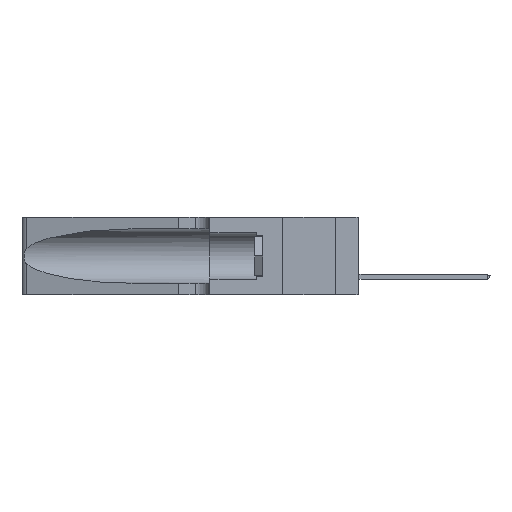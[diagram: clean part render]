
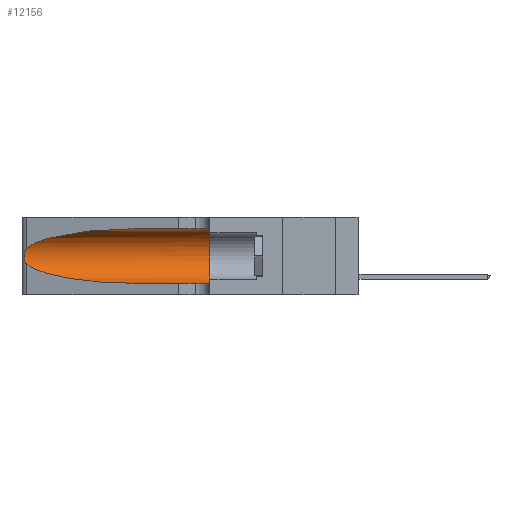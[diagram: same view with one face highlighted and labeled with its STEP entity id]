
A CAD part, left-side view. The second image highlights one B-rep face of the part: STEP entity #12156.
In plain terms, the highlighted cylindrical face has radius 3.308 mm (diameter 6.617 mm), a partial arc.
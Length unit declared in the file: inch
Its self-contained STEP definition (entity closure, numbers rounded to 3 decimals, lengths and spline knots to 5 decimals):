
#287 = B_SPLINE_CURVE_WITH_KNOTS ( 'NONE', 3,
 ( #22355, #33885, #36813, #13155, #19237, #19104, #28234, #21798, #3859, #10048, #34020, #1123, #4136, #34168 ),
 .UNSPECIFIED., .F., .F.,
 ( 4, 2, 2, 2, 2, 2, 4 ),
 ( 0., 0.00027, 0.00053, 0.00107, 0.0016, 0.00187, 0.00214 ),
 .UNSPECIFIED. ) ;
#646 = EDGE_CURVE ( 'NONE', #30015, #37181, #14277, .T. ) ;
#689 = CARTESIAN_POINT ( 'NONE',  ( 0.1305, 0.72297, 0.31525 ) ) ;
#1123 = CARTESIAN_POINT ( 'NONE',  ( 0.25639, 1.23186, 0.15144 ) ) ;
#1220 = CARTESIAN_POINT ( 'NONE',  ( 0.1305, 1.61858, 0.185 ) ) ;
#1498 = CARTESIAN_POINT ( 'NONE',  ( 0.1305, 1.61858, 0.31525 ) ) ;
#2928 = EDGE_CURVE ( 'NONE', #7715, #30015, #287, .T. ) ;
#3859 = CARTESIAN_POINT ( 'NONE',  ( 0.26017, 1.23833, 0.17102 ) ) ;
#4136 = CARTESIAN_POINT ( 'NONE',  ( 0.25555, 1.22993, 0.14849 ) ) ;
#4545 = CARTESIAN_POINT ( 'NONE',  ( 0.1305, 0.72297, 0.05475 ) ) ;
#4835 = LINE ( 'NONE', #1498, #13749 ) ;
#5540 = VERTEX_POINT ( 'NONE', #19862 ) ;
#5572 = VECTOR ( 'NONE', #37356, 39.37008 ) ;
#5904 = CARTESIAN_POINT ( 'NONE',  ( 0.25487, 1.22718, 0.22369 ) ) ;
#6229 = CARTESIAN_POINT ( 'NONE',  ( 0.25487, 1.22718, 0.14631 ) ) ;
#6385 = AXIS2_PLACEMENT_3D ( 'NONE', #1220, #34538, #34395 ) ;
#7013 = CARTESIAN_POINT ( 'NONE',  ( 0.25487, 1.22718, 0.22369 ) ) ;
#7155 = CARTESIAN_POINT ( 'NONE',  ( 0.2373, 1.15595, 0.28018 ) ) ;
#7715 = VERTEX_POINT ( 'NONE', #5904 ) ;
#8183 = ORIENTED_EDGE ( 'NONE', *, *, #2928, .T. ) ;
#8356 = CYLINDRICAL_SURFACE ( 'NONE', #6385, 0.13025 ) ;
#9649 = FACE_OUTER_BOUND ( 'NONE', #17999, .T. ) ;
#10024 = DIRECTION ( 'NONE',  ( 0., -1., 0. ) ) ;
#10048 = CARTESIAN_POINT ( 'NONE',  ( 0.25856, 1.23593, 0.16098 ) ) ;
#10107 = CARTESIAN_POINT ( 'NONE',  ( 0.1305, 0.35, 0.185 ) ) ;
#10376 = DIRECTION ( 'NONE',  ( 0., 1., 0. ) ) ;
#10422 = EDGE_CURVE ( 'NONE', #11902, #5540, #28086, .T. ) ;
#10718 = CARTESIAN_POINT ( 'NONE',  ( 0.2373, 1.15595, 0.08982 ) ) ;
#11196 = CARTESIAN_POINT ( 'NONE',  ( 0.1305, 0.72297, 0.05475 ) ) ;
#11902 = VERTEX_POINT ( 'NONE', #19878 ) ;
#12156 = ADVANCED_FACE ( 'NONE', ( #9649 ), #8356, .F. ) ;
#13155 = CARTESIAN_POINT ( 'NONE',  ( 0.25787, 1.23484, 0.2124 ) ) ;
#13441 = ORIENTED_EDGE ( 'NONE', *, *, #10422, .F. ) ;
#13749 = VECTOR ( 'NONE', #10024, 39.37008 ) ;
#14277 =( BOUNDED_CURVE ( )  B_SPLINE_CURVE ( 3, ( #31507, #10718, #31638, #4545 ),
 .UNSPECIFIED., .F., .T. ) 
 B_SPLINE_CURVE_WITH_KNOTS ( ( 4, 4 ),
 ( 3.44316, 4.71239 ),
 .UNSPECIFIED. ) 
 CURVE ( )  GEOMETRIC_REPRESENTATION_ITEM ( )  RATIONAL_B_SPLINE_CURVE ( ( 1., 0.87, 0.87, 1. ) ) 
 REPRESENTATION_ITEM ( '' )  );
#15396 =( BOUNDED_CURVE ( )  B_SPLINE_CURVE ( 3, ( #689, #18948, #7155, #7013 ),
 .UNSPECIFIED., .F., .T. ) 
 B_SPLINE_CURVE_WITH_KNOTS ( ( 4, 4 ),
 ( 1.5708, 2.84003 ),
 .UNSPECIFIED. ) 
 CURVE ( )  GEOMETRIC_REPRESENTATION_ITEM ( )  RATIONAL_B_SPLINE_CURVE ( ( 1., 0.87, 0.87, 1. ) ) 
 REPRESENTATION_ITEM ( '' )  );
#16196 = VERTEX_POINT ( 'NONE', #25013 ) ;
#16547 = EDGE_CURVE ( 'NONE', #37181, #5540, #37481, .T. ) ;
#16785 = EDGE_CURVE ( 'NONE', #16196, #7715, #15396, .T. ) ;
#17999 = EDGE_LOOP ( 'NONE', ( #30331, #8183, #38618, #18238, #13441, #19939 ) ) ;
#18238 = ORIENTED_EDGE ( 'NONE', *, *, #16547, .T. ) ;
#18948 = CARTESIAN_POINT ( 'NONE',  ( 0.18966, 0.96281, 0.31525 ) ) ;
#19104 = CARTESIAN_POINT ( 'NONE',  ( 0.26018, 1.23835, 0.19895 ) ) ;
#19237 = CARTESIAN_POINT ( 'NONE',  ( 0.25854, 1.2359, 0.20912 ) ) ;
#19862 = CARTESIAN_POINT ( 'NONE',  ( 0.1305, 0.35, 0.05475 ) ) ;
#19878 = CARTESIAN_POINT ( 'NONE',  ( 0.1305, 0.35, 0.31525 ) ) ;
#19939 = ORIENTED_EDGE ( 'NONE', *, *, #29448, .F. ) ;
#21798 = CARTESIAN_POINT ( 'NONE',  ( 0.26075, 1.23896, 0.178 ) ) ;
#22355 = CARTESIAN_POINT ( 'NONE',  ( 0.25487, 1.22718, 0.22369 ) ) ;
#25013 = CARTESIAN_POINT ( 'NONE',  ( 0.1305, 0.72297, 0.31525 ) ) ;
#26909 = CARTESIAN_POINT ( 'NONE',  ( 0.1305, 1.61858, 0.05475 ) ) ;
#28005 = DIRECTION ( 'NONE',  ( 0., 0., 1. ) ) ;
#28086 = CIRCLE ( 'NONE', #33191, 0.13025 ) ;
#28234 = CARTESIAN_POINT ( 'NONE',  ( 0.26075, 1.23896, 0.19203 ) ) ;
#29448 = EDGE_CURVE ( 'NONE', #16196, #11902, #4835, .T. ) ;
#30015 = VERTEX_POINT ( 'NONE', #6229 ) ;
#30331 = ORIENTED_EDGE ( 'NONE', *, *, #16785, .T. ) ;
#31507 = CARTESIAN_POINT ( 'NONE',  ( 0.25487, 1.22718, 0.14631 ) ) ;
#31638 = CARTESIAN_POINT ( 'NONE',  ( 0.18966, 0.96281, 0.05475 ) ) ;
#33191 = AXIS2_PLACEMENT_3D ( 'NONE', #10107, #10376, #28005 ) ;
#33885 = CARTESIAN_POINT ( 'NONE',  ( 0.25555, 1.22994, 0.2215 ) ) ;
#34020 = CARTESIAN_POINT ( 'NONE',  ( 0.25789, 1.23486, 0.15765 ) ) ;
#34168 = CARTESIAN_POINT ( 'NONE',  ( 0.25487, 1.22718, 0.14631 ) ) ;
#34395 = DIRECTION ( 'NONE',  ( 0., 0., -1. ) ) ;
#34538 = DIRECTION ( 'NONE',  ( 0., -1., 0. ) ) ;
#36813 = CARTESIAN_POINT ( 'NONE',  ( 0.25639, 1.23184, 0.21858 ) ) ;
#37181 = VERTEX_POINT ( 'NONE', #11196 ) ;
#37356 = DIRECTION ( 'NONE',  ( 0., -1., 0. ) ) ;
#37481 = LINE ( 'NONE', #26909, #5572 ) ;
#38618 = ORIENTED_EDGE ( 'NONE', *, *, #646, .T. ) ;
